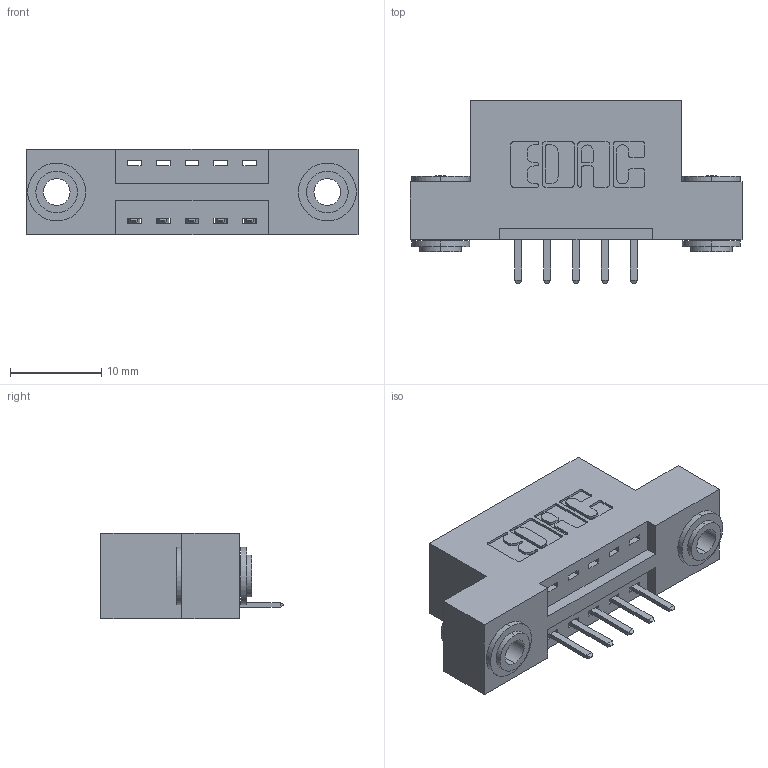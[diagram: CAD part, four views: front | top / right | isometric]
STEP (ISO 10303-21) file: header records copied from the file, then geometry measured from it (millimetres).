
FILE_DESCRIPTION (( 'STEP AP203' ), '1' );
FILE_NAME ('346-005-520-103.STEP', '2022-05-04T17:24:12', ( '' ), ( '' ), 'SwSTEP 2.0', 'SolidWorks 2020', '' );
FILE_SCHEMA (( 'CONFIG_CONTROL_DESIGN' ));
Length unit declared in the file: inch
Products named in the file (4): 345-292-001_345-293-120; 346 Part_Flush Mounting Lugs - 0.156 Dia-TH; 345-250-002_345-250-002-102; 346-005-520-103
Assembly tree (8 placements, depth 2):
  346-005-520-103
    346 Part_Flush Mounting Lugs - 0.156 Dia-TH
    345-292-001_345-293-120  x5
    345-250-002_345-250-002-102  x2
Bounding box: 36.45 x 20.02 x 9.4 mm (x, y, z)
Volume: 3221 mm3; surface area: 3830 mm2
Topology: 8 solids, 8 shells, 484 faces, 1361 edges, 890 vertices
Faces by surface type: plane 310, cylinder 166, cone 8
Entity records: 9264 total; most frequent: CARTESIAN_POINT 1592, ORIENTED_EDGE 1510, DIRECTION 1467, EDGE_CURVE 755, VECTOR 575, LINE 575, VERTEX_POINT 498, AXIS2_PLACEMENT_3D 446
